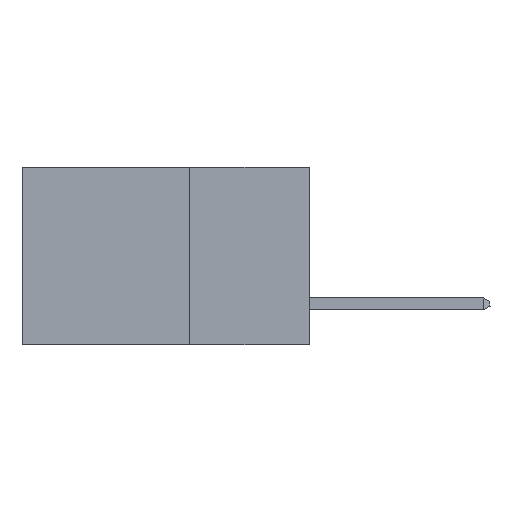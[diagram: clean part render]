
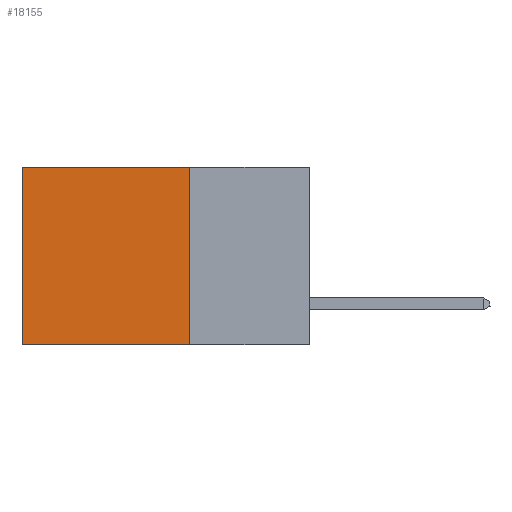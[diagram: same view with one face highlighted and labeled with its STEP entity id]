
A CAD part, left-side view. The second image highlights one B-rep face of the part: STEP entity #18155.
In plain terms, the highlighted planar face has unit normal (-1, 0, 0).
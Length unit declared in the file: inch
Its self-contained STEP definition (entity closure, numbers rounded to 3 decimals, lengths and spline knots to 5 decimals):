
#111 = CARTESIAN_POINT ( 'NONE',  ( 0.2875, 0.6, -0.37 ) ) ;
#1044 = EDGE_CURVE ( 'NONE', #4748, #5141, #4529, .T. ) ;
#2555 = DIRECTION ( 'NONE',  ( 0., 1., 0. ) ) ;
#2774 = CARTESIAN_POINT ( 'NONE',  ( 0.2875, 0.25, 0. ) ) ;
#2974 = VERTEX_POINT ( 'NONE', #111 ) ;
#3154 = EDGE_CURVE ( 'NONE', #4748, #15001, #12562, .T. ) ;
#3849 = CARTESIAN_POINT ( 'NONE',  ( 0.2875, 0.6, 0. ) ) ;
#4178 = VECTOR ( 'NONE', #10544, 39.37008 ) ;
#4529 = LINE ( 'NONE', #2774, #20381 ) ;
#4748 = VERTEX_POINT ( 'NONE', #11936 ) ;
#5141 = VERTEX_POINT ( 'NONE', #20292 ) ;
#5787 = FACE_OUTER_BOUND ( 'NONE', #6961, .T. ) ;
#6961 = EDGE_LOOP ( 'NONE', ( #14074, #18440, #17336, #17689 ) ) ;
#8898 = EDGE_CURVE ( 'NONE', #15001, #2974, #17922, .T. ) ;
#10510 = LINE ( 'NONE', #13108, #17925 ) ;
#10544 = DIRECTION ( 'NONE',  ( 0., 1., 0. ) ) ;
#10846 = AXIS2_PLACEMENT_3D ( 'NONE', #19134, #11023, #10969 ) ;
#10969 = DIRECTION ( 'NONE',  ( 0., 0., -1. ) ) ;
#11023 = DIRECTION ( 'NONE',  ( 1., 0., 0. ) ) ;
#11936 = CARTESIAN_POINT ( 'NONE',  ( 0.2875, 0.25, 0. ) ) ;
#12057 = CARTESIAN_POINT ( 'NONE',  ( 0.2875, 0.25, 0. ) ) ;
#12562 = LINE ( 'NONE', #12057, #4178 ) ;
#12802 = PLANE ( 'NONE',  #10846 ) ;
#13108 = CARTESIAN_POINT ( 'NONE',  ( 0.2875, 0.25, -0.37 ) ) ;
#13233 = DIRECTION ( 'NONE',  ( 0., 0., -1. ) ) ;
#13479 = VECTOR ( 'NONE', #13233, 39.37008 ) ;
#14074 = ORIENTED_EDGE ( 'NONE', *, *, #8898, .T. ) ;
#15001 = VERTEX_POINT ( 'NONE', #18841 ) ;
#15472 = DIRECTION ( 'NONE',  ( 0., 0., -1. ) ) ;
#17336 = ORIENTED_EDGE ( 'NONE', *, *, #1044, .F. ) ;
#17689 = ORIENTED_EDGE ( 'NONE', *, *, #3154, .T. ) ;
#17814 = EDGE_CURVE ( 'NONE', #5141, #2974, #10510, .T. ) ;
#17922 = LINE ( 'NONE', #3849, #13479 ) ;
#17925 = VECTOR ( 'NONE', #2555, 39.37008 ) ;
#18155 = ADVANCED_FACE ( 'NONE', ( #5787 ), #12802, .F. ) ;
#18440 = ORIENTED_EDGE ( 'NONE', *, *, #17814, .F. ) ;
#18841 = CARTESIAN_POINT ( 'NONE',  ( 0.2875, 0.6, 0. ) ) ;
#19134 = CARTESIAN_POINT ( 'NONE',  ( 0.2875, 0.25, 0. ) ) ;
#20292 = CARTESIAN_POINT ( 'NONE',  ( 0.2875, 0.25, -0.37 ) ) ;
#20381 = VECTOR ( 'NONE', #15472, 39.37008 ) ;
